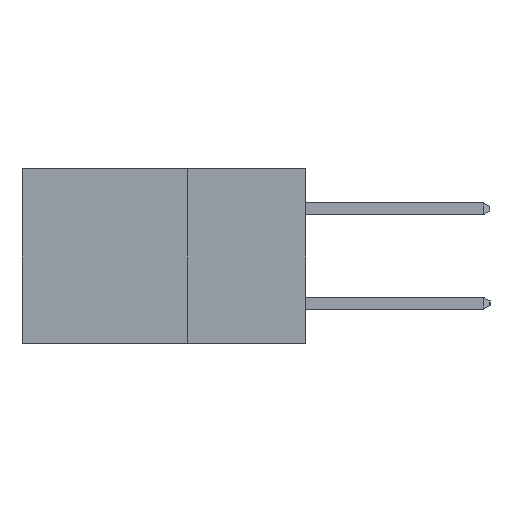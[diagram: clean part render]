
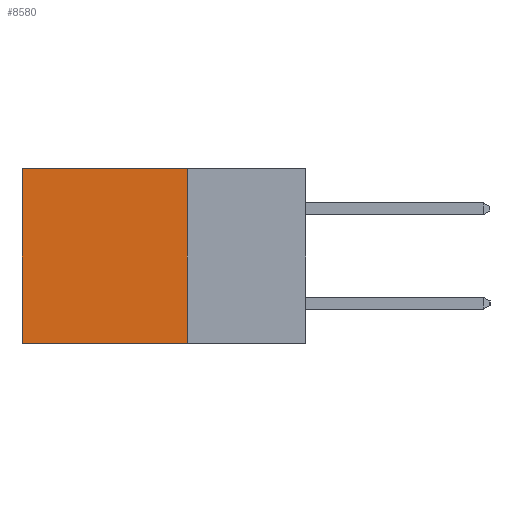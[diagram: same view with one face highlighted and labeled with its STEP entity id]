
A CAD part, left-side view. The second image highlights one B-rep face of the part: STEP entity #8580.
In plain terms, the highlighted planar face has unit normal (-1, 0, 0).
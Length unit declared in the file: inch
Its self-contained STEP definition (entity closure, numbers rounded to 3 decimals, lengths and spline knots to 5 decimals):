
#244 = CARTESIAN_POINT ( 'NONE',  ( 0.2615, 0.6, -0.37 ) ) ;
#637 = VECTOR ( 'NONE', #12250, 39.37008 ) ;
#1515 = EDGE_LOOP ( 'NONE', ( #15902, #14983, #12913, #18182 ) ) ;
#3122 = VERTEX_POINT ( 'NONE', #5737 ) ;
#3773 = DIRECTION ( 'NONE',  ( 0., 0., -1. ) ) ;
#4258 = VECTOR ( 'NONE', #3773, 39.37008 ) ;
#5588 = EDGE_CURVE ( 'NONE', #18801, #18784, #12647, .T. ) ;
#5737 = CARTESIAN_POINT ( 'NONE',  ( 0.2615, 0.25, -0.37 ) ) ;
#5881 = EDGE_CURVE ( 'NONE', #3122, #18784, #11468, .T. ) ;
#6203 = DIRECTION ( 'NONE',  ( 1., 0., 0. ) ) ;
#6945 = AXIS2_PLACEMENT_3D ( 'NONE', #11978, #6203, #16488 ) ;
#8397 = CARTESIAN_POINT ( 'NONE',  ( 0.2615, 0.25, -0.37 ) ) ;
#8580 = ADVANCED_FACE ( 'NONE', ( #18140 ), #15020, .F. ) ;
#9169 = DIRECTION ( 'NONE',  ( 0., 0., -1. ) ) ;
#9214 = CARTESIAN_POINT ( 'NONE',  ( 0.2615, 0.6, 0. ) ) ;
#9422 = CARTESIAN_POINT ( 'NONE',  ( 0.2615, 0.25, -0.37 ) ) ;
#9568 = CARTESIAN_POINT ( 'NONE',  ( 0.2615, 0.25, 0. ) ) ;
#9853 = DIRECTION ( 'NONE',  ( 0., 1., 0. ) ) ;
#10785 = CARTESIAN_POINT ( 'NONE',  ( 0.2615, 0.25, 0. ) ) ;
#11284 = VERTEX_POINT ( 'NONE', #9568 ) ;
#11468 = LINE ( 'NONE', #8397, #18735 ) ;
#11978 = CARTESIAN_POINT ( 'NONE',  ( 0.2615, 0.25, -0.37 ) ) ;
#12250 = DIRECTION ( 'NONE',  ( 0., 1., 0. ) ) ;
#12432 = LINE ( 'NONE', #10785, #637 ) ;
#12647 = LINE ( 'NONE', #17892, #16565 ) ;
#12913 = ORIENTED_EDGE ( 'NONE', *, *, #17085, .F. ) ;
#14907 = EDGE_CURVE ( 'NONE', #11284, #18801, #12432, .T. ) ;
#14983 = ORIENTED_EDGE ( 'NONE', *, *, #5881, .F. ) ;
#15020 = PLANE ( 'NONE',  #6945 ) ;
#15902 = ORIENTED_EDGE ( 'NONE', *, *, #5588, .T. ) ;
#16029 = LINE ( 'NONE', #9422, #4258 ) ;
#16488 = DIRECTION ( 'NONE',  ( 0., 0., -1. ) ) ;
#16565 = VECTOR ( 'NONE', #9169, 39.37008 ) ;
#17085 = EDGE_CURVE ( 'NONE', #11284, #3122, #16029, .T. ) ;
#17892 = CARTESIAN_POINT ( 'NONE',  ( 0.2615, 0.6, -0.37 ) ) ;
#18140 = FACE_OUTER_BOUND ( 'NONE', #1515, .T. ) ;
#18182 = ORIENTED_EDGE ( 'NONE', *, *, #14907, .T. ) ;
#18735 = VECTOR ( 'NONE', #9853, 39.37008 ) ;
#18784 = VERTEX_POINT ( 'NONE', #244 ) ;
#18801 = VERTEX_POINT ( 'NONE', #9214 ) ;
